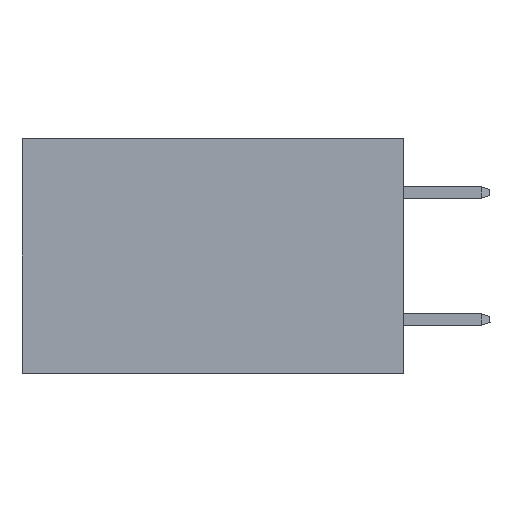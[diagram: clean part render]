
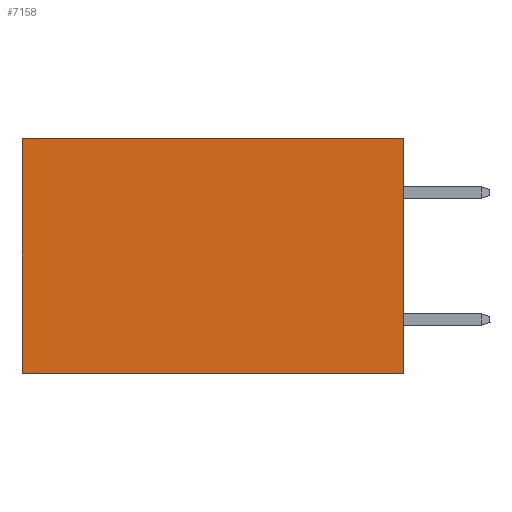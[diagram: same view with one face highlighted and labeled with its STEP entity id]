
A CAD part, left-side view. The second image highlights one B-rep face of the part: STEP entity #7158.
In plain terms, the highlighted planar face has unit normal (-1, 0, 0).
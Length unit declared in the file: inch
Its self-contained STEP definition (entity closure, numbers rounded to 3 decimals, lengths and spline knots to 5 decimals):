
#379 = EDGE_CURVE ( 'NONE', #11233, #20144, #4746, .T. ) ;
#1024 = VECTOR ( 'NONE', #16230, 39.37008 ) ;
#1668 = CARTESIAN_POINT ( 'NONE',  ( 0.2875, 0.6, 0. ) ) ;
#2770 = CARTESIAN_POINT ( 'NONE',  ( 0.2875, 0., 0. ) ) ;
#3868 = LINE ( 'NONE', #7164, #8886 ) ;
#4251 = CARTESIAN_POINT ( 'NONE',  ( 0.2875, 0., -0.37 ) ) ;
#4314 = DIRECTION ( 'NONE',  ( 0., 0., -1. ) ) ;
#4746 = LINE ( 'NONE', #11223, #6390 ) ;
#6267 = DIRECTION ( 'NONE',  ( 1., 0., 0. ) ) ;
#6390 = VECTOR ( 'NONE', #17954, 39.37008 ) ;
#6635 = DIRECTION ( 'NONE',  ( 0., 0., -1. ) ) ;
#7158 = ADVANCED_FACE ( 'NONE', ( #12860 ), #21346, .F. ) ;
#7164 = CARTESIAN_POINT ( 'NONE',  ( 0.2875, 0.6, 0. ) ) ;
#7717 = DIRECTION ( 'NONE',  ( 0., 0., -1. ) ) ;
#8161 = EDGE_CURVE ( 'NONE', #9290, #16356, #9515, .T. ) ;
#8886 = VECTOR ( 'NONE', #6635, 39.37008 ) ;
#9290 = VERTEX_POINT ( 'NONE', #20645 ) ;
#9515 = LINE ( 'NONE', #4251, #1024 ) ;
#10338 = EDGE_CURVE ( 'NONE', #11233, #9290, #14198, .T. ) ;
#11223 = CARTESIAN_POINT ( 'NONE',  ( 0.2875, 0., 0. ) ) ;
#11233 = VERTEX_POINT ( 'NONE', #14779 ) ;
#12860 = FACE_OUTER_BOUND ( 'NONE', #21332, .T. ) ;
#14198 = LINE ( 'NONE', #16086, #18704 ) ;
#14314 = ORIENTED_EDGE ( 'NONE', *, *, #10338, .F. ) ;
#14779 = CARTESIAN_POINT ( 'NONE',  ( 0.2875, 0., 0. ) ) ;
#16072 = AXIS2_PLACEMENT_3D ( 'NONE', #2770, #6267, #4314 ) ;
#16086 = CARTESIAN_POINT ( 'NONE',  ( 0.2875, 0., 0. ) ) ;
#16230 = DIRECTION ( 'NONE',  ( 0., 1., 0. ) ) ;
#16356 = VERTEX_POINT ( 'NONE', #17422 ) ;
#17422 = CARTESIAN_POINT ( 'NONE',  ( 0.2875, 0.6, -0.37 ) ) ;
#17954 = DIRECTION ( 'NONE',  ( 0., 1., 0. ) ) ;
#18140 = EDGE_CURVE ( 'NONE', #20144, #16356, #3868, .T. ) ;
#18704 = VECTOR ( 'NONE', #7717, 39.37008 ) ;
#20057 = ORIENTED_EDGE ( 'NONE', *, *, #18140, .T. ) ;
#20144 = VERTEX_POINT ( 'NONE', #1668 ) ;
#20158 = ORIENTED_EDGE ( 'NONE', *, *, #8161, .F. ) ;
#20607 = ORIENTED_EDGE ( 'NONE', *, *, #379, .T. ) ;
#20645 = CARTESIAN_POINT ( 'NONE',  ( 0.2875, 0., -0.37 ) ) ;
#21332 = EDGE_LOOP ( 'NONE', ( #20057, #20158, #14314, #20607 ) ) ;
#21346 = PLANE ( 'NONE',  #16072 ) ;
